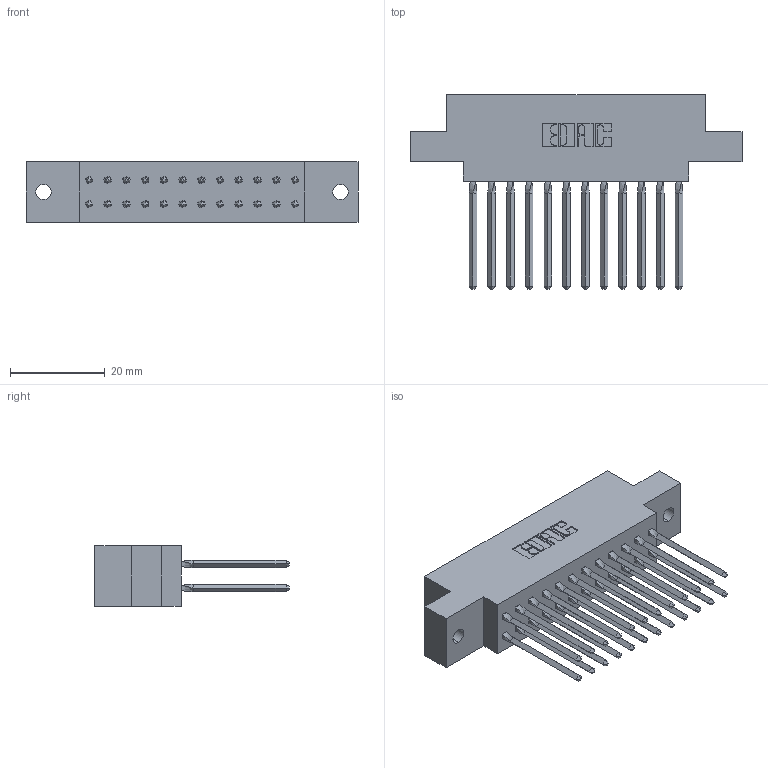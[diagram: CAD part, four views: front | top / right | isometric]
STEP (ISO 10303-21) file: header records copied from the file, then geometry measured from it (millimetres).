
FILE_DESCRIPTION (( 'STEP AP203' ), '1' );
FILE_NAME ('317-024-543-802.STEP', '2020-02-27T18:16:17', ( '' ), ( '' ), 'SwSTEP 2.0', 'SolidWorks 2016', '' );
FILE_SCHEMA (( 'CONFIG_CONTROL_DESIGN' ));
Length unit declared in the file: inch
Products named in the file (3): 317-024-543-802; 317 Part_.144 Dia; 317-290-001_543
Assembly tree (25 placements, depth 2):
  317-024-543-802
    317 Part_.144 Dia
    317-290-001_543  x24
Bounding box: 70.26 x 41.15 x 12.7 mm (x, y, z)
Volume: 10859.6 mm3; surface area: 15033.9 mm2
Topology: 25 solids, 25 shells, 2238 faces, 6203 edges, 3998 vertices
Faces by surface type: plane 1810, cylinder 332, bspline 96
Entity records: 21534 total; most frequent: CARTESIAN_POINT 4167, ORIENTED_EDGE 3666, DIRECTION 3063, EDGE_CURVE 1833, VECTOR 1577, LINE 1577, VERTEX_POINT 1215, AXIS2_PLACEMENT_3D 743
